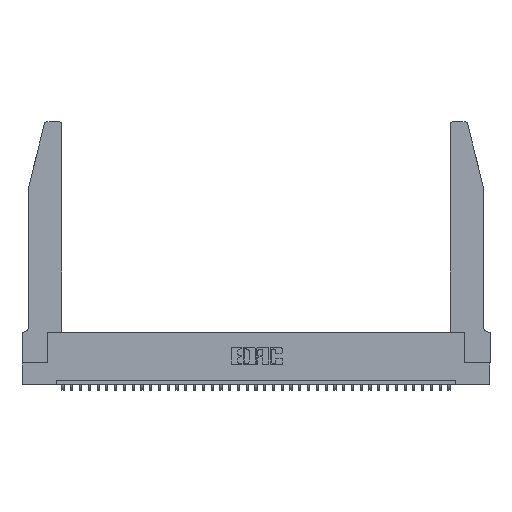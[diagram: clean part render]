
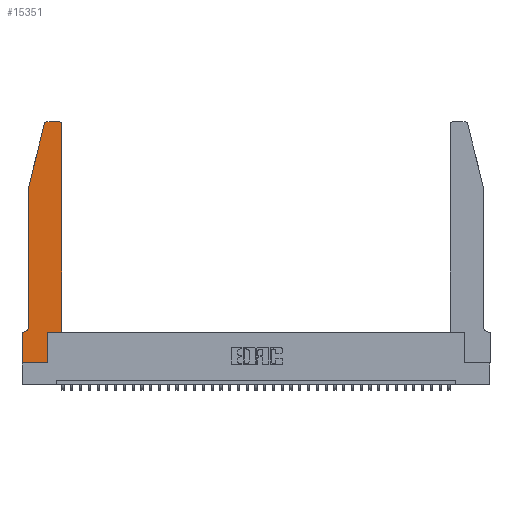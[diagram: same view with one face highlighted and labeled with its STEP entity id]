
A CAD part, top view. The second image highlights one B-rep face of the part: STEP entity #15351.
In plain terms, the highlighted planar face has unit normal (0, 0, 1).
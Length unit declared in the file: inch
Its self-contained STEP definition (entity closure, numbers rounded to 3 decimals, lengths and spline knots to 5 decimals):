
#817 = FACE_OUTER_BOUND ( 'NONE', #35836, .T. ) ;
#1398 = EDGE_CURVE ( 'NONE', #26038, #1989, #12353, .T. ) ;
#1528 = VERTEX_POINT ( 'NONE', #28879 ) ;
#1989 = VERTEX_POINT ( 'NONE', #7364 ) ;
#2194 = ORIENTED_EDGE ( 'NONE', *, *, #9655, .T. ) ;
#2453 = CARTESIAN_POINT ( 'NONE',  ( 0.0755, 0.35, 0.37 ) ) ;
#2974 = PLANE ( 'NONE',  #7640 ) ;
#3134 = DIRECTION ( 'NONE',  ( 0., 1., 0. ) ) ;
#3559 = VERTEX_POINT ( 'NONE', #13022 ) ;
#4635 = CARTESIAN_POINT ( 'NONE',  ( 0.0755, 2., 0.37 ) ) ;
#6673 = ORIENTED_EDGE ( 'NONE', *, *, #20312, .T. ) ;
#6728 = CARTESIAN_POINT ( 'NONE',  ( 0., 0., 0.37 ) ) ;
#7110 = VERTEX_POINT ( 'NONE', #34110 ) ;
#7364 = CARTESIAN_POINT ( 'NONE',  ( 0.2865, 0., 0.37 ) ) ;
#7640 = AXIS2_PLACEMENT_3D ( 'NONE', #17865, #20806, #18474 ) ;
#8266 = VERTEX_POINT ( 'NONE', #19068 ) ;
#8498 = EDGE_CURVE ( 'NONE', #26763, #16277, #9116, .T. ) ;
#8558 = LINE ( 'NONE', #34458, #31193 ) ;
#8950 = VERTEX_POINT ( 'NONE', #35303 ) ;
#9116 = CIRCLE ( 'NONE', #21291, 0.03 ) ;
#9655 = EDGE_CURVE ( 'NONE', #1989, #7110, #12226, .T. ) ;
#10869 = DIRECTION ( 'NONE',  ( -0.239, -0.971, 0. ) ) ;
#10890 = LINE ( 'NONE', #19506, #31689 ) ;
#10906 = CARTESIAN_POINT ( 'NONE',  ( 0., 0., 0.37 ) ) ;
#11163 = CARTESIAN_POINT ( 'NONE',  ( 0.4505, 0.35, 0.37 ) ) ;
#11817 = VECTOR ( 'NONE', #16862, 39.37008 ) ;
#12023 = DIRECTION ( 'NONE',  ( 0., -1., 0. ) ) ;
#12199 = LINE ( 'NONE', #4635, #36233 ) ;
#12226 = LINE ( 'NONE', #30965, #18255 ) ;
#12258 = CARTESIAN_POINT ( 'NONE',  ( 0.0055, 0.42, 0.37 ) ) ;
#12353 = LINE ( 'NONE', #18940, #19308 ) ;
#12503 = DIRECTION ( 'NONE',  ( -1., 0., 0. ) ) ;
#12905 = EDGE_CURVE ( 'NONE', #26758, #26763, #15707, .T. ) ;
#13022 = CARTESIAN_POINT ( 'NONE',  ( 0.0755, 2., 0.37 ) ) ;
#13298 = CARTESIAN_POINT ( 'NONE',  ( 0.284, 2.75, 0.37 ) ) ;
#13552 = DIRECTION ( 'NONE',  ( 1., 0., 0. ) ) ;
#13919 = CARTESIAN_POINT ( 'NONE',  ( 0., 0.35, 0.37 ) ) ;
#14567 = LINE ( 'NONE', #2453, #24659 ) ;
#15351 = ADVANCED_FACE ( 'NONE', ( #817 ), #2974, .T. ) ;
#15707 = LINE ( 'NONE', #11163, #22168 ) ;
#15982 = EDGE_CURVE ( 'NONE', #16277, #20903, #16080, .T. ) ;
#16080 = LINE ( 'NONE', #29274, #32310 ) ;
#16277 = VERTEX_POINT ( 'NONE', #17557 ) ;
#16826 = AXIS2_PLACEMENT_3D ( 'NONE', #29413, #38171, #38040 ) ;
#16862 = DIRECTION ( 'NONE',  ( 0., -1., 0. ) ) ;
#17091 = DIRECTION ( 'NONE',  ( -1., 0., 0. ) ) ;
#17557 = CARTESIAN_POINT ( 'NONE',  ( 0.4205, 2.75, 0.37 ) ) ;
#17583 = DIRECTION ( 'NONE',  ( 1., 0., 0. ) ) ;
#17785 = CIRCLE ( 'NONE', #29337, 0.07 ) ;
#17865 = CARTESIAN_POINT ( 'NONE',  ( 0., 0.35, 0.37 ) ) ;
#18255 = VECTOR ( 'NONE', #3134, 39.37008 ) ;
#18474 = DIRECTION ( 'NONE',  ( 1., 0., 0. ) ) ;
#18597 = EDGE_CURVE ( 'NONE', #3559, #8266, #8558, .T. ) ;
#18940 = CARTESIAN_POINT ( 'NONE',  ( 0., 0., 0.37 ) ) ;
#19068 = CARTESIAN_POINT ( 'NONE',  ( 0.0755, 0.42, 0.37 ) ) ;
#19137 = ORIENTED_EDGE ( 'NONE', *, *, #1398, .T. ) ;
#19308 = VECTOR ( 'NONE', #31077, 39.37008 ) ;
#19431 = ORIENTED_EDGE ( 'NONE', *, *, #20243, .T. ) ;
#19506 = CARTESIAN_POINT ( 'NONE',  ( 0.4505, 0.35, 0.37 ) ) ;
#19981 = EDGE_CURVE ( 'NONE', #24763, #26038, #25632, .T. ) ;
#20243 = EDGE_CURVE ( 'NONE', #7110, #26758, #10890, .T. ) ;
#20312 = EDGE_CURVE ( 'NONE', #8950, #3559, #12199, .T. ) ;
#20353 = EDGE_CURVE ( 'NONE', #1528, #24763, #14567, .T. ) ;
#20462 = ORIENTED_EDGE ( 'NONE', *, *, #8498, .T. ) ;
#20806 = DIRECTION ( 'NONE',  ( 0., 0., 1. ) ) ;
#20903 = VERTEX_POINT ( 'NONE', #13298 ) ;
#21291 = AXIS2_PLACEMENT_3D ( 'NONE', #38313, #35624, #17583 ) ;
#22168 = VECTOR ( 'NONE', #34915, 39.37008 ) ;
#22229 = ORIENTED_EDGE ( 'NONE', *, *, #15982, .T. ) ;
#24028 = CARTESIAN_POINT ( 'NONE',  ( 0.4505, 2.72, 0.37 ) ) ;
#24659 = VECTOR ( 'NONE', #17091, 39.37008 ) ;
#24748 = CIRCLE ( 'NONE', #16826, 0.03 ) ;
#24763 = VERTEX_POINT ( 'NONE', #13919 ) ;
#25632 = LINE ( 'NONE', #10906, #11817 ) ;
#25915 = ORIENTED_EDGE ( 'NONE', *, *, #12905, .T. ) ;
#25925 = ORIENTED_EDGE ( 'NONE', *, *, #19981, .T. ) ;
#26038 = VERTEX_POINT ( 'NONE', #6728 ) ;
#26202 = ORIENTED_EDGE ( 'NONE', *, *, #18597, .T. ) ;
#26758 = VERTEX_POINT ( 'NONE', #32852 ) ;
#26763 = VERTEX_POINT ( 'NONE', #24028 ) ;
#28879 = CARTESIAN_POINT ( 'NONE',  ( 0.0055, 0.35, 0.37 ) ) ;
#29270 = ORIENTED_EDGE ( 'NONE', *, *, #29775, .T. ) ;
#29274 = CARTESIAN_POINT ( 'NONE',  ( 0.2605, 2.75, 0.37 ) ) ;
#29337 = AXIS2_PLACEMENT_3D ( 'NONE', #12258, #32949, #12503 ) ;
#29413 = CARTESIAN_POINT ( 'NONE',  ( 0.284, 2.72, 0.37 ) ) ;
#29775 = EDGE_CURVE ( 'NONE', #8266, #1528, #17785, .T. ) ;
#30965 = CARTESIAN_POINT ( 'NONE',  ( 0.2865, 0.35, 0.37 ) ) ;
#31077 = DIRECTION ( 'NONE',  ( 1., 0., 0. ) ) ;
#31193 = VECTOR ( 'NONE', #12023, 39.37008 ) ;
#31689 = VECTOR ( 'NONE', #13552, 39.37008 ) ;
#32310 = VECTOR ( 'NONE', #35450, 39.37008 ) ;
#32852 = CARTESIAN_POINT ( 'NONE',  ( 0.4505, 0.35, 0.37 ) ) ;
#32949 = DIRECTION ( 'NONE',  ( 0., 0., -1. ) ) ;
#33831 = ORIENTED_EDGE ( 'NONE', *, *, #35367, .T. ) ;
#34110 = CARTESIAN_POINT ( 'NONE',  ( 0.2865, 0.35, 0.37 ) ) ;
#34458 = CARTESIAN_POINT ( 'NONE',  ( 0.0755, 2., 0.37 ) ) ;
#34915 = DIRECTION ( 'NONE',  ( 0., 1., 0. ) ) ;
#35303 = CARTESIAN_POINT ( 'NONE',  ( 0.25487, 2.72718, 0.37 ) ) ;
#35367 = EDGE_CURVE ( 'NONE', #20903, #8950, #24748, .T. ) ;
#35450 = DIRECTION ( 'NONE',  ( -1., 0., 0. ) ) ;
#35624 = DIRECTION ( 'NONE',  ( 0., 0., 1. ) ) ;
#35836 = EDGE_LOOP ( 'NONE', ( #22229, #33831, #6673, #26202, #29270, #36333, #25925, #19137, #2194, #19431, #25915, #20462 ) ) ;
#36233 = VECTOR ( 'NONE', #10869, 39.37008 ) ;
#36333 = ORIENTED_EDGE ( 'NONE', *, *, #20353, .T. ) ;
#38040 = DIRECTION ( 'NONE',  ( 1., 0., 0. ) ) ;
#38171 = DIRECTION ( 'NONE',  ( 0., 0., 1. ) ) ;
#38313 = CARTESIAN_POINT ( 'NONE',  ( 0.4205, 2.72, 0.37 ) ) ;
